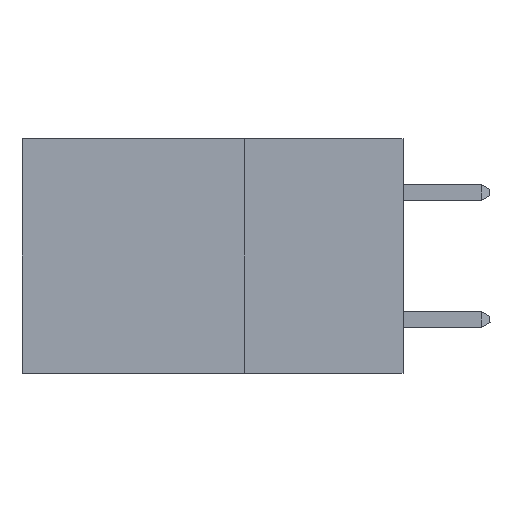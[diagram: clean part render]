
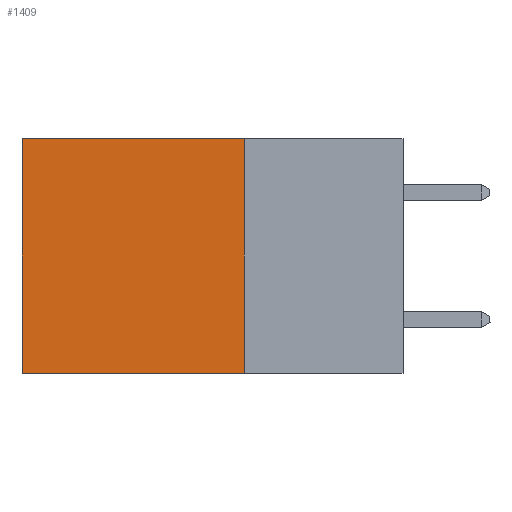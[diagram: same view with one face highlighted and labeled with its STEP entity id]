
A CAD part, left-side view. The second image highlights one B-rep face of the part: STEP entity #1409.
In plain terms, the highlighted planar face has unit normal (-1, 0, 0).
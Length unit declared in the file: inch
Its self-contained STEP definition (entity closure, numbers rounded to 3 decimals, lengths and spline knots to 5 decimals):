
#769 = CARTESIAN_POINT ( 'NONE',  ( 0.2875, 0.6, 0. ) ) ;
#1047 = VERTEX_POINT ( 'NONE', #6808 ) ;
#1146 = VECTOR ( 'NONE', #9254, 39.37008 ) ;
#1159 = EDGE_CURVE ( 'NONE', #1617, #1047, #2758, .T. ) ;
#1341 = DIRECTION ( 'NONE',  ( 0., 1., 0. ) ) ;
#1409 = ADVANCED_FACE ( 'NONE', ( #8676 ), #10726, .F. ) ;
#1425 = DIRECTION ( 'NONE',  ( 0., 0., -1. ) ) ;
#1617 = VERTEX_POINT ( 'NONE', #1837 ) ;
#1675 = VERTEX_POINT ( 'NONE', #4527 ) ;
#1837 = CARTESIAN_POINT ( 'NONE',  ( 0.2875, 0.6, 0. ) ) ;
#2477 = EDGE_CURVE ( 'NONE', #1675, #6806, #9693, .T. ) ;
#2758 = LINE ( 'NONE', #769, #1146 ) ;
#2787 = VECTOR ( 'NONE', #3878, 39.37008 ) ;
#3028 = DIRECTION ( 'NONE',  ( 1., 0., 0. ) ) ;
#3878 = DIRECTION ( 'NONE',  ( 0., 1., 0. ) ) ;
#4527 = CARTESIAN_POINT ( 'NONE',  ( 0.2875, 0.25, 0. ) ) ;
#4687 = AXIS2_PLACEMENT_3D ( 'NONE', #8734, #3028, #11681 ) ;
#4908 = LINE ( 'NONE', #9771, #10113 ) ;
#6505 = ORIENTED_EDGE ( 'NONE', *, *, #11147, .T. ) ;
#6806 = VERTEX_POINT ( 'NONE', #10480 ) ;
#6808 = CARTESIAN_POINT ( 'NONE',  ( 0.2875, 0.6, -0.37 ) ) ;
#7531 = ORIENTED_EDGE ( 'NONE', *, *, #2477, .F. ) ;
#8366 = VECTOR ( 'NONE', #1425, 39.37008 ) ;
#8637 = EDGE_CURVE ( 'NONE', #6806, #1047, #4908, .T. ) ;
#8675 = EDGE_LOOP ( 'NONE', ( #9368, #12056, #7531, #6505 ) ) ;
#8676 = FACE_OUTER_BOUND ( 'NONE', #8675, .T. ) ;
#8734 = CARTESIAN_POINT ( 'NONE',  ( 0.2875, 0.25, 0. ) ) ;
#9254 = DIRECTION ( 'NONE',  ( 0., 0., -1. ) ) ;
#9368 = ORIENTED_EDGE ( 'NONE', *, *, #1159, .T. ) ;
#9693 = LINE ( 'NONE', #10875, #8366 ) ;
#9771 = CARTESIAN_POINT ( 'NONE',  ( 0.2875, 0.25, -0.37 ) ) ;
#10113 = VECTOR ( 'NONE', #1341, 39.37008 ) ;
#10353 = LINE ( 'NONE', #10543, #2787 ) ;
#10480 = CARTESIAN_POINT ( 'NONE',  ( 0.2875, 0.25, -0.37 ) ) ;
#10543 = CARTESIAN_POINT ( 'NONE',  ( 0.2875, 0.25, 0. ) ) ;
#10726 = PLANE ( 'NONE',  #4687 ) ;
#10875 = CARTESIAN_POINT ( 'NONE',  ( 0.2875, 0.25, 0. ) ) ;
#11147 = EDGE_CURVE ( 'NONE', #1675, #1617, #10353, .T. ) ;
#11681 = DIRECTION ( 'NONE',  ( 0., 0., -1. ) ) ;
#12056 = ORIENTED_EDGE ( 'NONE', *, *, #8637, .F. ) ;
